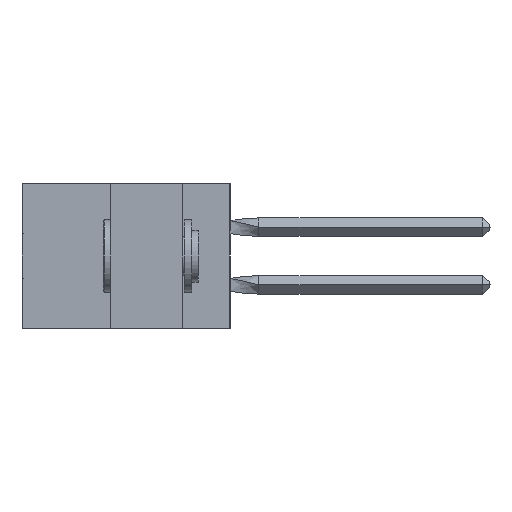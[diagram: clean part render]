
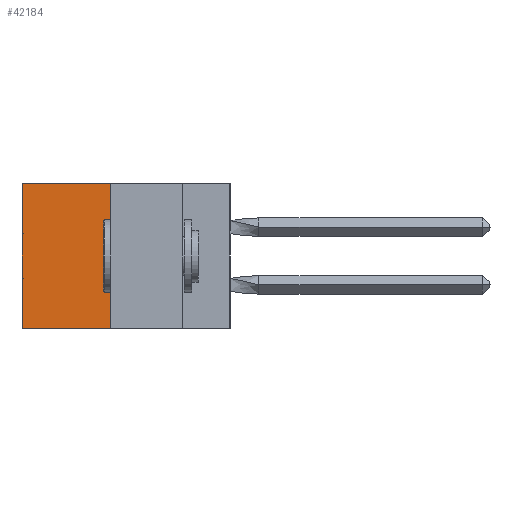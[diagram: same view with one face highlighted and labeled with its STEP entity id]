
A CAD part, left-side view. The second image highlights one B-rep face of the part: STEP entity #42184.
In plain terms, the highlighted planar face has unit normal (-1, 0, 0).
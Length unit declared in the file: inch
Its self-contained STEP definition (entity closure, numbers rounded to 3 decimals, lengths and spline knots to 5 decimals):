
#2576 = PLANE ( 'NONE',  #32344 ) ;
#7313 = CARTESIAN_POINT ( 'NONE',  ( 0.305, 0.413, 0. ) ) ;
#7432 = EDGE_CURVE ( 'NONE', #8145, #19463, #37130, .T. ) ;
#8145 = VERTEX_POINT ( 'NONE', #7313 ) ;
#8710 = ORIENTED_EDGE ( 'NONE', *, *, #33690, .T. ) ;
#9523 = EDGE_LOOP ( 'NONE', ( #41440, #13895, #42541, #8710 ) ) ;
#9999 = VERTEX_POINT ( 'NONE', #42935 ) ;
#10036 = CARTESIAN_POINT ( 'NONE',  ( 0.305, 0.413, 0. ) ) ;
#10715 = CARTESIAN_POINT ( 'NONE',  ( 0.305, 0.413, -0.5 ) ) ;
#12106 = EDGE_CURVE ( 'NONE', #9999, #12340, #43853, .T. ) ;
#12340 = VERTEX_POINT ( 'NONE', #16524 ) ;
#13895 = ORIENTED_EDGE ( 'NONE', *, *, #35020, .F. ) ;
#14521 = DIRECTION ( 'NONE',  ( 0., 0., -1. ) ) ;
#15738 = FACE_OUTER_BOUND ( 'NONE', #9523, .T. ) ;
#16524 = CARTESIAN_POINT ( 'NONE',  ( 0.305, 0.72, -0.5 ) ) ;
#19328 = LINE ( 'NONE', #10036, #29476 ) ;
#19463 = VERTEX_POINT ( 'NONE', #24966 ) ;
#19871 = VECTOR ( 'NONE', #46073, 39.37008 ) ;
#21820 = DIRECTION ( 'NONE',  ( 0., 0., -1. ) ) ;
#24966 = CARTESIAN_POINT ( 'NONE',  ( 0.305, 0.413, -0.5 ) ) ;
#24999 = DIRECTION ( 'NONE',  ( 1., 0., 0. ) ) ;
#25244 = VECTOR ( 'NONE', #46208, 39.37008 ) ;
#29476 = VECTOR ( 'NONE', #36725, 39.37008 ) ;
#30578 = LINE ( 'NONE', #40775, #19871 ) ;
#31086 = VECTOR ( 'NONE', #14521, 39.37008 ) ;
#32344 = AXIS2_PLACEMENT_3D ( 'NONE', #44752, #24999, #21820 ) ;
#33690 = EDGE_CURVE ( 'NONE', #8145, #9999, #19328, .T. ) ;
#34459 = CARTESIAN_POINT ( 'NONE',  ( 0.305, 0.72, -0.5 ) ) ;
#35020 = EDGE_CURVE ( 'NONE', #19463, #12340, #30578, .T. ) ;
#36725 = DIRECTION ( 'NONE',  ( 0., 1., 0. ) ) ;
#37130 = LINE ( 'NONE', #10715, #31086 ) ;
#40775 = CARTESIAN_POINT ( 'NONE',  ( 0.305, 0.413, -0.5 ) ) ;
#41440 = ORIENTED_EDGE ( 'NONE', *, *, #12106, .T. ) ;
#42184 = ADVANCED_FACE ( 'NONE', ( #15738 ), #2576, .F. ) ;
#42541 = ORIENTED_EDGE ( 'NONE', *, *, #7432, .F. ) ;
#42935 = CARTESIAN_POINT ( 'NONE',  ( 0.305, 0.72, 0. ) ) ;
#43853 = LINE ( 'NONE', #34459, #25244 ) ;
#44752 = CARTESIAN_POINT ( 'NONE',  ( 0.305, 0.413, -0.5 ) ) ;
#46073 = DIRECTION ( 'NONE',  ( 0., 1., 0. ) ) ;
#46208 = DIRECTION ( 'NONE',  ( 0., 0., -1. ) ) ;
